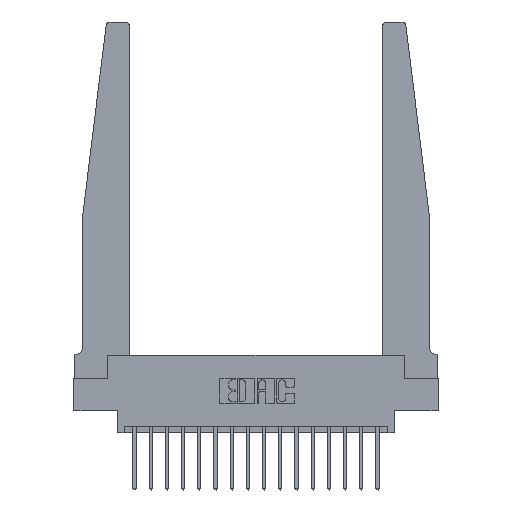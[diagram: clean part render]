
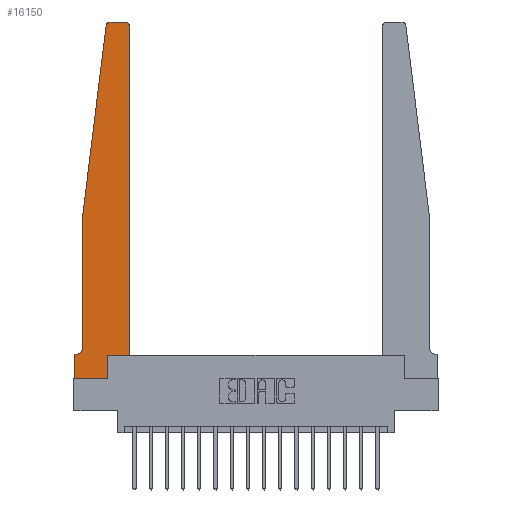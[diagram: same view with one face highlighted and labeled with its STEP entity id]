
A CAD part, top view. The second image highlights one B-rep face of the part: STEP entity #16150.
In plain terms, the highlighted planar face has unit normal (0, 0, 1).
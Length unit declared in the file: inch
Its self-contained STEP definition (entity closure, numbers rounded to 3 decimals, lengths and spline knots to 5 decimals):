
#13 = VECTOR ( 'NONE', #5265, 39.37008 ) ;
#152 = CARTESIAN_POINT ( 'NONE',  ( 0.425, 0.18, 0.37 ) ) ;
#243 = ORIENTED_EDGE ( 'NONE', *, *, #777, .T. ) ;
#489 = EDGE_CURVE ( 'NONE', #16560, #11689, #11622, .T. ) ;
#544 = VECTOR ( 'NONE', #5880, 39.37008 ) ;
#559 = CARTESIAN_POINT ( 'NONE',  ( 0.015, 0.2375, 0.37 ) ) ;
#692 = AXIS2_PLACEMENT_3D ( 'NONE', #8405, #12900, #11413 ) ;
#777 = EDGE_CURVE ( 'NONE', #18971, #4767, #13143, .T. ) ;
#948 = EDGE_CURVE ( 'NONE', #3227, #18949, #13613, .T. ) ;
#1195 = ORIENTED_EDGE ( 'NONE', *, *, #489, .T. ) ;
#1262 = LINE ( 'NONE', #7311, #7819 ) ;
#1354 = DIRECTION ( 'NONE',  ( 0., 0., 1. ) ) ;
#1675 = VECTOR ( 'NONE', #13707, 39.37008 ) ;
#1826 = CARTESIAN_POINT ( 'NONE',  ( 0., 0., 0.37 ) ) ;
#1896 = EDGE_CURVE ( 'NONE', #11689, #18971, #2617, .T. ) ;
#2045 = VECTOR ( 'NONE', #7393, 39.37008 ) ;
#2060 = EDGE_CURVE ( 'NONE', #18949, #4473, #3074, .T. ) ;
#2455 = VERTEX_POINT ( 'NONE', #4243 ) ;
#2617 = LINE ( 'NONE', #15955, #13254 ) ;
#2761 = CARTESIAN_POINT ( 'NONE',  ( 0.065, 1.25, 0.37 ) ) ;
#3074 = LINE ( 'NONE', #152, #2045 ) ;
#3200 = AXIS2_PLACEMENT_3D ( 'NONE', #559, #6214, #14122 ) ;
#3227 = VERTEX_POINT ( 'NONE', #6839 ) ;
#3961 = DIRECTION ( 'NONE',  ( 1., 0., 0. ) ) ;
#4016 = VERTEX_POINT ( 'NONE', #11033 ) ;
#4221 = CARTESIAN_POINT ( 'NONE',  ( 0.2605, 0.18, 0.37 ) ) ;
#4243 = CARTESIAN_POINT ( 'NONE',  ( 0.2605, 0., 0.37 ) ) ;
#4280 = DIRECTION ( 'NONE',  ( -1., 0., 0. ) ) ;
#4473 = VERTEX_POINT ( 'NONE', #13053 ) ;
#4534 = ORIENTED_EDGE ( 'NONE', *, *, #12729, .T. ) ;
#4767 = VERTEX_POINT ( 'NONE', #1826 ) ;
#4903 = ORIENTED_EDGE ( 'NONE', *, *, #17613, .T. ) ;
#5244 = CARTESIAN_POINT ( 'NONE',  ( 0.425, 0.18, 0.37 ) ) ;
#5265 = DIRECTION ( 'NONE',  ( 0., -1., 0. ) ) ;
#5474 = EDGE_CURVE ( 'NONE', #14277, #6740, #9107, .T. ) ;
#5608 = VECTOR ( 'NONE', #3961, 39.37008 ) ;
#5686 = LINE ( 'NONE', #4221, #16468 ) ;
#5880 = DIRECTION ( 'NONE',  ( -0.122, -0.992, 0. ) ) ;
#5924 = DIRECTION ( 'NONE',  ( 0., 0., 1. ) ) ;
#6099 = CARTESIAN_POINT ( 'NONE',  ( 0., 0., 0.37 ) ) ;
#6214 = DIRECTION ( 'NONE',  ( 0., 0., -1. ) ) ;
#6740 = VERTEX_POINT ( 'NONE', #7761 ) ;
#6839 = CARTESIAN_POINT ( 'NONE',  ( 0.2605, 0.18, 0.37 ) ) ;
#6967 = VECTOR ( 'NONE', #14791, 39.37008 ) ;
#7279 = EDGE_CURVE ( 'NONE', #8809, #14277, #1262, .T. ) ;
#7309 = DIRECTION ( 'NONE',  ( 1., 0., 0. ) ) ;
#7311 = CARTESIAN_POINT ( 'NONE',  ( 0.25, 2.75, 0.37 ) ) ;
#7393 = DIRECTION ( 'NONE',  ( 0., 1., 0. ) ) ;
#7761 = CARTESIAN_POINT ( 'NONE',  ( 0.24675, 2.72367, 0.37 ) ) ;
#7819 = VECTOR ( 'NONE', #4280, 39.37008 ) ;
#8165 = CARTESIAN_POINT ( 'NONE',  ( 0.015, 0.1875, 0.37 ) ) ;
#8222 = ORIENTED_EDGE ( 'NONE', *, *, #7279, .T. ) ;
#8405 = CARTESIAN_POINT ( 'NONE',  ( 0.27653, 2.72, 0.37 ) ) ;
#8473 = DIRECTION ( 'NONE',  ( -1., 0., 0. ) ) ;
#8809 = VERTEX_POINT ( 'NONE', #14212 ) ;
#8943 = CARTESIAN_POINT ( 'NONE',  ( 0., 0.1875, 0.37 ) ) ;
#8984 = ORIENTED_EDGE ( 'NONE', *, *, #1896, .T. ) ;
#9107 = CIRCLE ( 'NONE', #692, 0.03 ) ;
#9532 = LINE ( 'NONE', #9729, #5608 ) ;
#9619 = DIRECTION ( 'NONE',  ( 0., 1., 0. ) ) ;
#9729 = CARTESIAN_POINT ( 'NONE',  ( 0., 0., 0.37 ) ) ;
#9883 = ORIENTED_EDGE ( 'NONE', *, *, #2060, .T. ) ;
#10266 = LINE ( 'NONE', #2761, #544 ) ;
#10684 = CARTESIAN_POINT ( 'NONE',  ( 0.425, 0.18, 0.37 ) ) ;
#11033 = CARTESIAN_POINT ( 'NONE',  ( 0.065, 1.25, 0.37 ) ) ;
#11392 = LINE ( 'NONE', #12675, #13 ) ;
#11413 = DIRECTION ( 'NONE',  ( 1., 0., 0. ) ) ;
#11622 = CIRCLE ( 'NONE', #3200, 0.05 ) ;
#11689 = VERTEX_POINT ( 'NONE', #8165 ) ;
#11815 = CARTESIAN_POINT ( 'NONE',  ( 0.065, 0.2375, 0.37 ) ) ;
#12104 = ORIENTED_EDGE ( 'NONE', *, *, #5474, .T. ) ;
#12222 = EDGE_CURVE ( 'NONE', #6740, #4016, #10266, .T. ) ;
#12607 = EDGE_CURVE ( 'NONE', #4016, #16560, #11392, .T. ) ;
#12675 = CARTESIAN_POINT ( 'NONE',  ( 0.065, 1.25, 0.37 ) ) ;
#12729 = EDGE_CURVE ( 'NONE', #4473, #8809, #17799, .T. ) ;
#12900 = DIRECTION ( 'NONE',  ( 0., 0., 1. ) ) ;
#13053 = CARTESIAN_POINT ( 'NONE',  ( 0.425, 2.72, 0.37 ) ) ;
#13143 = LINE ( 'NONE', #6099, #6967 ) ;
#13254 = VECTOR ( 'NONE', #8473, 39.37008 ) ;
#13434 = DIRECTION ( 'NONE',  ( 1., 0., 0. ) ) ;
#13613 = LINE ( 'NONE', #10684, #1675 ) ;
#13707 = DIRECTION ( 'NONE',  ( 1., 0., 0. ) ) ;
#13988 = AXIS2_PLACEMENT_3D ( 'NONE', #19016, #5924, #13434 ) ;
#14122 = DIRECTION ( 'NONE',  ( -1., 0., 0. ) ) ;
#14127 = ORIENTED_EDGE ( 'NONE', *, *, #12607, .T. ) ;
#14212 = CARTESIAN_POINT ( 'NONE',  ( 0.395, 2.75, 0.37 ) ) ;
#14277 = VERTEX_POINT ( 'NONE', #15453 ) ;
#14683 = AXIS2_PLACEMENT_3D ( 'NONE', #14714, #1354, #7309 ) ;
#14714 = CARTESIAN_POINT ( 'NONE',  ( 0.395, 2.72, 0.37 ) ) ;
#14791 = DIRECTION ( 'NONE',  ( 0., -1., 0. ) ) ;
#15055 = ORIENTED_EDGE ( 'NONE', *, *, #16515, .T. ) ;
#15453 = CARTESIAN_POINT ( 'NONE',  ( 0.27653, 2.75, 0.37 ) ) ;
#15955 = CARTESIAN_POINT ( 'NONE',  ( 0.065, 0.1875, 0.37 ) ) ;
#16108 = ORIENTED_EDGE ( 'NONE', *, *, #12222, .T. ) ;
#16148 = PLANE ( 'NONE',  #13988 ) ;
#16150 = ADVANCED_FACE ( 'NONE', ( #17268 ), #16148, .T. ) ;
#16468 = VECTOR ( 'NONE', #9619, 39.37008 ) ;
#16485 = EDGE_LOOP ( 'NONE', ( #8222, #12104, #16108, #14127, #1195, #8984, #243, #4903, #15055, #17507, #9883, #4534 ) ) ;
#16515 = EDGE_CURVE ( 'NONE', #2455, #3227, #5686, .T. ) ;
#16560 = VERTEX_POINT ( 'NONE', #11815 ) ;
#17268 = FACE_OUTER_BOUND ( 'NONE', #16485, .T. ) ;
#17507 = ORIENTED_EDGE ( 'NONE', *, *, #948, .T. ) ;
#17613 = EDGE_CURVE ( 'NONE', #4767, #2455, #9532, .T. ) ;
#17799 = CIRCLE ( 'NONE', #14683, 0.03 ) ;
#18949 = VERTEX_POINT ( 'NONE', #5244 ) ;
#18971 = VERTEX_POINT ( 'NONE', #8943 ) ;
#19016 = CARTESIAN_POINT ( 'NONE',  ( 0., 0.1875, 0.37 ) ) ;
